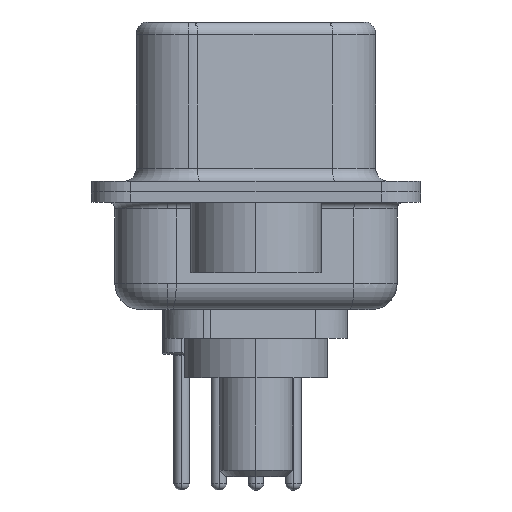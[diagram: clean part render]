
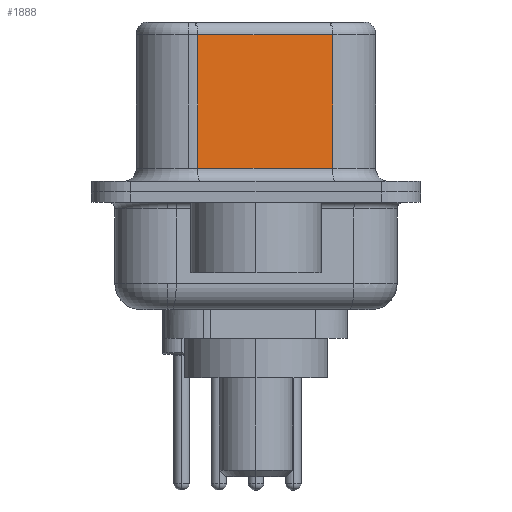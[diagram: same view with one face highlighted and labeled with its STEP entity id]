
A CAD part, left-side view. The second image highlights one B-rep face of the part: STEP entity #1888.
In plain terms, the highlighted planar face has unit normal (-0.985, -0.174, 0).
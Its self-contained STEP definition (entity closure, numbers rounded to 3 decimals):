
#121 = CARTESIAN_POINT ( 'NONE',  ( 4.58, -2.927, 6.02 ) ) ;
#999 = EDGE_CURVE ( 'NONE', #17920, #16644, #2893, .T. ) ;
#1291 = EDGE_CURVE ( 'NONE', #19436, #6888, #15165, .T. ) ;
#1888 = ADVANCED_FACE ( 'NONE', ( #6226 ), #6985, .F. ) ;
#2281 = ORIENTED_EDGE ( 'NONE', *, *, #11076, .F. ) ;
#2893 = LINE ( 'NONE', #22011, #16594 ) ;
#4375 = CARTESIAN_POINT ( 'NONE',  ( 4.58, -2.927, 6.52 ) ) ;
#4600 = EDGE_CURVE ( 'NONE', #6888, #17920, #8188, .T. ) ;
#5182 = DIRECTION ( 'NONE',  ( 0.985, 0.174, 0. ) ) ;
#5324 = ORIENTED_EDGE ( 'NONE', *, *, #999, .T. ) ;
#5580 = DIRECTION ( 'NONE',  ( -0.174, 0.985, 0. ) ) ;
#5625 = VECTOR ( 'NONE', #22041, 1000. ) ;
#6205 = ORIENTED_EDGE ( 'NONE', *, *, #4600, .T. ) ;
#6226 = FACE_OUTER_BOUND ( 'NONE', #22774, .T. ) ;
#6457 = ORIENTED_EDGE ( 'NONE', *, *, #1291, .T. ) ;
#6760 = LINE ( 'NONE', #4375, #5625 ) ;
#6888 = VERTEX_POINT ( 'NONE', #20815 ) ;
#6985 = PLANE ( 'NONE',  #17387 ) ;
#7777 = CARTESIAN_POINT ( 'NONE',  ( 4.58, -2.927, 6.52 ) ) ;
#8188 = LINE ( 'NONE', #13497, #16526 ) ;
#9176 = CARTESIAN_POINT ( 'NONE',  ( 4.58, -2.927, 0.9 ) ) ;
#10410 = VECTOR ( 'NONE', #22271, 1000. ) ;
#11076 = EDGE_CURVE ( 'NONE', #19436, #16644, #6760, .T. ) ;
#13497 = CARTESIAN_POINT ( 'NONE',  ( 3.67, 2.233, 6.52 ) ) ;
#14217 = DIRECTION ( 'NONE',  ( 0., 0., -1. ) ) ;
#14923 = CARTESIAN_POINT ( 'NONE',  ( 3.67, 2.233, 0.9 ) ) ;
#15165 = LINE ( 'NONE', #15823, #10410 ) ;
#15823 = CARTESIAN_POINT ( 'NONE',  ( 4.58, -2.927, 6.02 ) ) ;
#16100 = DIRECTION ( 'NONE',  ( 0.174, -0.985, 0. ) ) ;
#16526 = VECTOR ( 'NONE', #14217, 1000. ) ;
#16594 = VECTOR ( 'NONE', #16100, 1000. ) ;
#16644 = VERTEX_POINT ( 'NONE', #9176 ) ;
#17387 = AXIS2_PLACEMENT_3D ( 'NONE', #7777, #5182, #5580 ) ;
#17920 = VERTEX_POINT ( 'NONE', #14923 ) ;
#19436 = VERTEX_POINT ( 'NONE', #121 ) ;
#20815 = CARTESIAN_POINT ( 'NONE',  ( 3.67, 2.233, 6.02 ) ) ;
#22011 = CARTESIAN_POINT ( 'NONE',  ( 4.58, -2.927, 0.9 ) ) ;
#22041 = DIRECTION ( 'NONE',  ( 0., 0., -1. ) ) ;
#22271 = DIRECTION ( 'NONE',  ( -0.174, 0.985, 0. ) ) ;
#22774 = EDGE_LOOP ( 'NONE', ( #2281, #6457, #6205, #5324 ) ) ;
